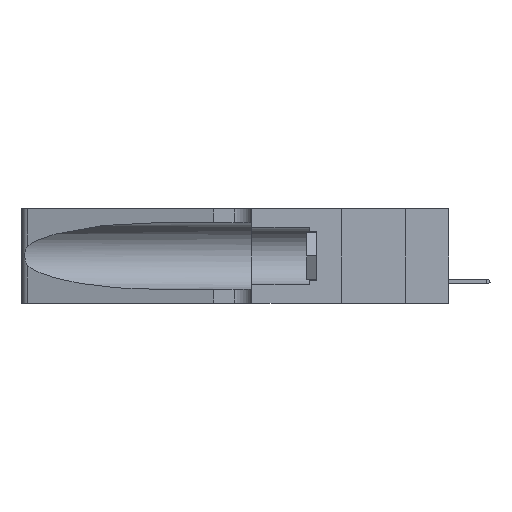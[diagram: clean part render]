
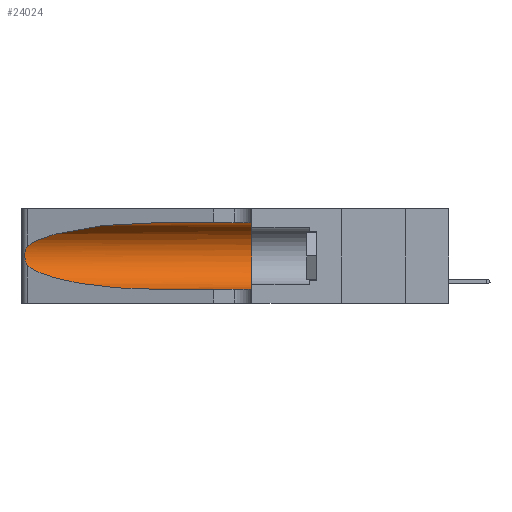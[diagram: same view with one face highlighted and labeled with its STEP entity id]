
A CAD part, left-side view. The second image highlights one B-rep face of the part: STEP entity #24024.
In plain terms, the highlighted cylindrical face has radius 3.308 mm (diameter 6.617 mm), a partial arc.
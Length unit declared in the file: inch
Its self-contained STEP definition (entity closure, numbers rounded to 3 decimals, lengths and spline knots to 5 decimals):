
#331 = EDGE_CURVE ( 'NONE', #27037, #33563, #30811, .T. ) ;
#1213 = CARTESIAN_POINT ( 'NONE',  ( 0.25555, 1.22994, 0.2215 ) ) ;
#1313 =( BOUNDED_CURVE ( )  B_SPLINE_CURVE ( 3, ( #7242, #10349, #32154, #32022 ),
 .UNSPECIFIED., .F., .T. ) 
 B_SPLINE_CURVE_WITH_KNOTS ( ( 4, 4 ),
 ( 3.44316, 4.71239 ),
 .UNSPECIFIED. ) 
 CURVE ( )  GEOMETRIC_REPRESENTATION_ITEM ( )  RATIONAL_B_SPLINE_CURVE ( ( 1., 0.87, 0.87, 1. ) ) 
 REPRESENTATION_ITEM ( '' )  );
#2769 = DIRECTION ( 'NONE',  ( 0., 0., 1. ) ) ;
#3069 = VERTEX_POINT ( 'NONE', #4796 ) ;
#3111 = ORIENTED_EDGE ( 'NONE', *, *, #8968, .T. ) ;
#4338 = CARTESIAN_POINT ( 'NONE',  ( 0.25639, 1.23184, 0.21858 ) ) ;
#4369 = VERTEX_POINT ( 'NONE', #17660 ) ;
#4796 = CARTESIAN_POINT ( 'NONE',  ( 0.25487, 1.22718, 0.14631 ) ) ;
#6258 = CARTESIAN_POINT ( 'NONE',  ( 0.1305, 0.35, 0.05475 ) ) ;
#6259 = B_SPLINE_CURVE_WITH_KNOTS ( 'NONE', 3,
 ( #7039, #1213, #4338, #38072, #13109, #10419, #32225, #7563, #35039, #26002, #16354, #34768, #22525, #7431 ),
 .UNSPECIFIED., .F., .F.,
 ( 4, 2, 2, 2, 2, 2, 4 ),
 ( 0., 0.00027, 0.00053, 0.00107, 0.0016, 0.00187, 0.00214 ),
 .UNSPECIFIED. ) ;
#6775 = EDGE_CURVE ( 'NONE', #9406, #6801, #25815, .T. ) ;
#6801 = VERTEX_POINT ( 'NONE', #6258 ) ;
#7039 = CARTESIAN_POINT ( 'NONE',  ( 0.25487, 1.22718, 0.22369 ) ) ;
#7242 = CARTESIAN_POINT ( 'NONE',  ( 0.25487, 1.22718, 0.14631 ) ) ;
#7431 = CARTESIAN_POINT ( 'NONE',  ( 0.25487, 1.22718, 0.14631 ) ) ;
#7563 = CARTESIAN_POINT ( 'NONE',  ( 0.26075, 1.23896, 0.178 ) ) ;
#7992 = CARTESIAN_POINT ( 'NONE',  ( 0.2373, 1.15595, 0.28018 ) ) ;
#8177 = AXIS2_PLACEMENT_3D ( 'NONE', #32414, #32542, #13972 ) ;
#8968 = EDGE_CURVE ( 'NONE', #3069, #4369, #1313, .T. ) ;
#9098 = DIRECTION ( 'NONE',  ( 0., 1., 0. ) ) ;
#9406 = VERTEX_POINT ( 'NONE', #13634 ) ;
#9641 = CARTESIAN_POINT ( 'NONE',  ( 0.1305, 1.61858, 0.05475 ) ) ;
#10202 = EDGE_CURVE ( 'NONE', #33563, #3069, #6259, .T. ) ;
#10349 = CARTESIAN_POINT ( 'NONE',  ( 0.2373, 1.15595, 0.08982 ) ) ;
#10419 = CARTESIAN_POINT ( 'NONE',  ( 0.26018, 1.23835, 0.19895 ) ) ;
#10862 = VECTOR ( 'NONE', #34537, 39.37008 ) ;
#11215 = EDGE_CURVE ( 'NONE', #4369, #6801, #39515, .T. ) ;
#11325 = EDGE_LOOP ( 'NONE', ( #16115, #35924, #3111, #15879, #27101, #24980 ) ) ;
#13109 = CARTESIAN_POINT ( 'NONE',  ( 0.25854, 1.2359, 0.20912 ) ) ;
#13110 = CARTESIAN_POINT ( 'NONE',  ( 0.1305, 1.61858, 0.31525 ) ) ;
#13634 = CARTESIAN_POINT ( 'NONE',  ( 0.1305, 0.35, 0.31525 ) ) ;
#13956 = CARTESIAN_POINT ( 'NONE',  ( 0.1305, 0.72297, 0.31525 ) ) ;
#13972 = DIRECTION ( 'NONE',  ( 0., 0., -1. ) ) ;
#15193 = CARTESIAN_POINT ( 'NONE',  ( 0.1305, 0.35, 0.185 ) ) ;
#15879 = ORIENTED_EDGE ( 'NONE', *, *, #11215, .T. ) ;
#16115 = ORIENTED_EDGE ( 'NONE', *, *, #331, .T. ) ;
#16354 = CARTESIAN_POINT ( 'NONE',  ( 0.25789, 1.23486, 0.15765 ) ) ;
#17660 = CARTESIAN_POINT ( 'NONE',  ( 0.1305, 0.72297, 0.05475 ) ) ;
#19105 = CARTESIAN_POINT ( 'NONE',  ( 0.25487, 1.22718, 0.22369 ) ) ;
#20700 = EDGE_CURVE ( 'NONE', #27037, #9406, #34554, .T. ) ;
#22385 = DIRECTION ( 'NONE',  ( 0., -1., 0. ) ) ;
#22525 = CARTESIAN_POINT ( 'NONE',  ( 0.25555, 1.22993, 0.14849 ) ) ;
#24024 = ADVANCED_FACE ( 'NONE', ( #36451 ), #39865, .F. ) ;
#24980 = ORIENTED_EDGE ( 'NONE', *, *, #20700, .F. ) ;
#25815 = CIRCLE ( 'NONE', #39489, 0.13025 ) ;
#26002 = CARTESIAN_POINT ( 'NONE',  ( 0.25856, 1.23593, 0.16098 ) ) ;
#27037 = VERTEX_POINT ( 'NONE', #36752 ) ;
#27101 = ORIENTED_EDGE ( 'NONE', *, *, #6775, .F. ) ;
#30811 =( BOUNDED_CURVE ( )  B_SPLINE_CURVE ( 3, ( #13956, #35758, #7992, #32788 ),
 .UNSPECIFIED., .F., .F. ) 
 B_SPLINE_CURVE_WITH_KNOTS ( ( 4, 4 ),
 ( 1.5708, 2.84003 ),
 .UNSPECIFIED. ) 
 CURVE ( )  GEOMETRIC_REPRESENTATION_ITEM ( )  RATIONAL_B_SPLINE_CURVE ( ( 1., 0.87, 0.87, 1. ) ) 
 REPRESENTATION_ITEM ( '' )  );
#32022 = CARTESIAN_POINT ( 'NONE',  ( 0.1305, 0.72297, 0.05475 ) ) ;
#32154 = CARTESIAN_POINT ( 'NONE',  ( 0.18966, 0.96281, 0.05475 ) ) ;
#32225 = CARTESIAN_POINT ( 'NONE',  ( 0.26075, 1.23896, 0.19203 ) ) ;
#32414 = CARTESIAN_POINT ( 'NONE',  ( 0.1305, 1.61858, 0.185 ) ) ;
#32542 = DIRECTION ( 'NONE',  ( 0., -1., 0. ) ) ;
#32788 = CARTESIAN_POINT ( 'NONE',  ( 0.25487, 1.22718, 0.22369 ) ) ;
#33563 = VERTEX_POINT ( 'NONE', #19105 ) ;
#34537 = DIRECTION ( 'NONE',  ( 0., -1., 0. ) ) ;
#34554 = LINE ( 'NONE', #13110, #34850 ) ;
#34768 = CARTESIAN_POINT ( 'NONE',  ( 0.25639, 1.23186, 0.15144 ) ) ;
#34850 = VECTOR ( 'NONE', #22385, 39.37008 ) ;
#35039 = CARTESIAN_POINT ( 'NONE',  ( 0.26017, 1.23833, 0.17102 ) ) ;
#35758 = CARTESIAN_POINT ( 'NONE',  ( 0.18966, 0.96281, 0.31525 ) ) ;
#35924 = ORIENTED_EDGE ( 'NONE', *, *, #10202, .T. ) ;
#36451 = FACE_OUTER_BOUND ( 'NONE', #11325, .T. ) ;
#36752 = CARTESIAN_POINT ( 'NONE',  ( 0.1305, 0.72297, 0.31525 ) ) ;
#38072 = CARTESIAN_POINT ( 'NONE',  ( 0.25787, 1.23484, 0.2124 ) ) ;
#39489 = AXIS2_PLACEMENT_3D ( 'NONE', #15193, #9098, #2769 ) ;
#39515 = LINE ( 'NONE', #9641, #10862 ) ;
#39865 = CYLINDRICAL_SURFACE ( 'NONE', #8177, 0.13025 ) ;
